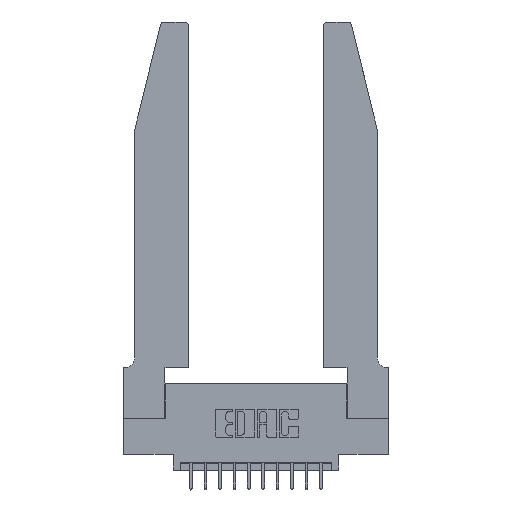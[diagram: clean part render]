
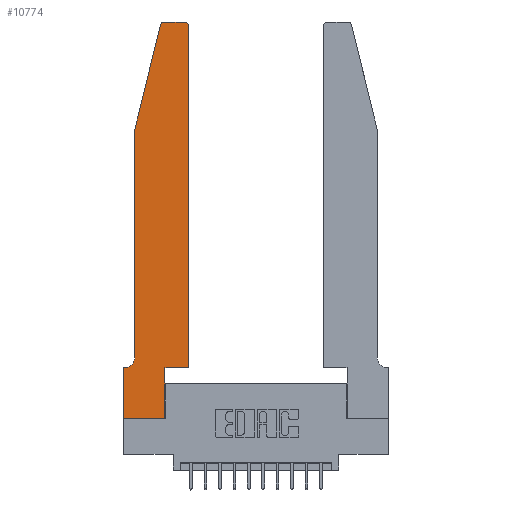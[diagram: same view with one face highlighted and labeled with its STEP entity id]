
A CAD part, top view. The second image highlights one B-rep face of the part: STEP entity #10774.
In plain terms, the highlighted planar face has unit normal (0, 0, 1).
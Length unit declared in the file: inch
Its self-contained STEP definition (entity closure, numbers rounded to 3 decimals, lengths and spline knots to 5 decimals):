
#90 = CARTESIAN_POINT ( 'NONE',  ( 0.0755, 2., 0.37 ) ) ;
#97 = CARTESIAN_POINT ( 'NONE',  ( 0.4505, 0.35, 0.37 ) ) ;
#165 = CIRCLE ( 'NONE', #15423, 0.07 ) ;
#335 = CARTESIAN_POINT ( 'NONE',  ( 0.0755, 0.42, 0.37 ) ) ;
#756 = VECTOR ( 'NONE', #4122, 39.37008 ) ;
#1157 = EDGE_CURVE ( 'NONE', #2570, #7950, #8377, .T. ) ;
#1395 = FACE_OUTER_BOUND ( 'NONE', #4094, .T. ) ;
#1536 = LINE ( 'NONE', #90, #12011 ) ;
#1605 = EDGE_CURVE ( 'NONE', #7950, #5005, #9120, .T. ) ;
#1927 = DIRECTION ( 'NONE',  ( 0., 0., -1. ) ) ;
#2083 = EDGE_CURVE ( 'NONE', #10482, #15649, #16942, .T. ) ;
#2090 = VERTEX_POINT ( 'NONE', #6530 ) ;
#2202 = AXIS2_PLACEMENT_3D ( 'NONE', #9430, #14817, #2800 ) ;
#2219 = CARTESIAN_POINT ( 'NONE',  ( 0.284, 2.75, 0.37 ) ) ;
#2226 = AXIS2_PLACEMENT_3D ( 'NONE', #7040, #16215, #12387 ) ;
#2570 = VERTEX_POINT ( 'NONE', #7397 ) ;
#2649 = CARTESIAN_POINT ( 'NONE',  ( 0.2605, 2.75, 0.37 ) ) ;
#2753 = VERTEX_POINT ( 'NONE', #16014 ) ;
#2800 = DIRECTION ( 'NONE',  ( 1., 0., 0. ) ) ;
#2968 = LINE ( 'NONE', #10841, #16239 ) ;
#3703 = AXIS2_PLACEMENT_3D ( 'NONE', #10741, #15989, #15657 ) ;
#3741 = ORIENTED_EDGE ( 'NONE', *, *, #15960, .T. ) ;
#3764 = VERTEX_POINT ( 'NONE', #15720 ) ;
#4094 = EDGE_LOOP ( 'NONE', ( #3741, #6626, #5440, #13302, #4902, #16029, #16630, #5879, #13497, #8921, #9785, #5282 ) ) ;
#4122 = DIRECTION ( 'NONE',  ( -1., 0., 0. ) ) ;
#4249 = VERTEX_POINT ( 'NONE', #335 ) ;
#4635 = CARTESIAN_POINT ( 'NONE',  ( 0., 0., 0.37 ) ) ;
#4716 = CIRCLE ( 'NONE', #2202, 0.03 ) ;
#4902 = ORIENTED_EDGE ( 'NONE', *, *, #15686, .T. ) ;
#5001 = LINE ( 'NONE', #10351, #11483 ) ;
#5005 = VERTEX_POINT ( 'NONE', #10716 ) ;
#5067 = CARTESIAN_POINT ( 'NONE',  ( 0.25487, 2.72718, 0.37 ) ) ;
#5282 = ORIENTED_EDGE ( 'NONE', *, *, #6026, .T. ) ;
#5380 = DIRECTION ( 'NONE',  ( 0., 1., 0. ) ) ;
#5440 = ORIENTED_EDGE ( 'NONE', *, *, #5965, .T. ) ;
#5478 = EDGE_CURVE ( 'NONE', #7269, #16284, #4716, .T. ) ;
#5767 = CARTESIAN_POINT ( 'NONE',  ( 0.2865, 0.35, 0.37 ) ) ;
#5879 = ORIENTED_EDGE ( 'NONE', *, *, #7337, .T. ) ;
#5965 = EDGE_CURVE ( 'NONE', #16284, #2090, #1536, .T. ) ;
#6026 = EDGE_CURVE ( 'NONE', #3764, #2753, #9749, .T. ) ;
#6442 = CARTESIAN_POINT ( 'NONE',  ( 0., 0., 0.37 ) ) ;
#6530 = CARTESIAN_POINT ( 'NONE',  ( 0.0755, 2., 0.37 ) ) ;
#6626 = ORIENTED_EDGE ( 'NONE', *, *, #5478, .T. ) ;
#7040 = CARTESIAN_POINT ( 'NONE',  ( 0.4205, 2.72, 0.37 ) ) ;
#7269 = VERTEX_POINT ( 'NONE', #2219 ) ;
#7337 = EDGE_CURVE ( 'NONE', #15649, #2570, #5001, .T. ) ;
#7397 = CARTESIAN_POINT ( 'NONE',  ( 0.2865, 0., 0.37 ) ) ;
#7950 = VERTEX_POINT ( 'NONE', #5767 ) ;
#8377 = LINE ( 'NONE', #13719, #16578 ) ;
#8412 = DIRECTION ( 'NONE',  ( -1., 0., 0. ) ) ;
#8921 = ORIENTED_EDGE ( 'NONE', *, *, #1605, .T. ) ;
#9120 = LINE ( 'NONE', #16748, #11090 ) ;
#9430 = CARTESIAN_POINT ( 'NONE',  ( 0.284, 2.72, 0.37 ) ) ;
#9749 = CIRCLE ( 'NONE', #2226, 0.03 ) ;
#9773 = CARTESIAN_POINT ( 'NONE',  ( 0.0055, 0.42, 0.37 ) ) ;
#9785 = ORIENTED_EDGE ( 'NONE', *, *, #14564, .T. ) ;
#10351 = CARTESIAN_POINT ( 'NONE',  ( 0., 0., 0.37 ) ) ;
#10473 = VECTOR ( 'NONE', #5380, 39.37008 ) ;
#10482 = VERTEX_POINT ( 'NONE', #14580 ) ;
#10716 = CARTESIAN_POINT ( 'NONE',  ( 0.4505, 0.35, 0.37 ) ) ;
#10741 = CARTESIAN_POINT ( 'NONE',  ( 0., 0.35, 0.37 ) ) ;
#10774 = ADVANCED_FACE ( 'NONE', ( #1395 ), #12069, .T. ) ;
#10786 = VERTEX_POINT ( 'NONE', #12240 ) ;
#10841 = CARTESIAN_POINT ( 'NONE',  ( 0.0755, 2., 0.37 ) ) ;
#11090 = VECTOR ( 'NONE', #12921, 39.37008 ) ;
#11272 = VECTOR ( 'NONE', #11799, 39.37008 ) ;
#11483 = VECTOR ( 'NONE', #14347, 39.37008 ) ;
#11799 = DIRECTION ( 'NONE',  ( 0., -1., 0. ) ) ;
#11956 = LINE ( 'NONE', #97, #10473 ) ;
#12011 = VECTOR ( 'NONE', #12216, 39.37008 ) ;
#12069 = PLANE ( 'NONE',  #3703 ) ;
#12216 = DIRECTION ( 'NONE',  ( -0.239, -0.971, 0. ) ) ;
#12240 = CARTESIAN_POINT ( 'NONE',  ( 0.0055, 0.35, 0.37 ) ) ;
#12387 = DIRECTION ( 'NONE',  ( 1., 0., 0. ) ) ;
#12539 = LINE ( 'NONE', #16544, #14882 ) ;
#12921 = DIRECTION ( 'NONE',  ( 1., 0., 0. ) ) ;
#13302 = ORIENTED_EDGE ( 'NONE', *, *, #15492, .T. ) ;
#13497 = ORIENTED_EDGE ( 'NONE', *, *, #1157, .T. ) ;
#13642 = DIRECTION ( 'NONE',  ( 0., -1., 0. ) ) ;
#13719 = CARTESIAN_POINT ( 'NONE',  ( 0.2865, 0.35, 0.37 ) ) ;
#14347 = DIRECTION ( 'NONE',  ( 1., 0., 0. ) ) ;
#14564 = EDGE_CURVE ( 'NONE', #5005, #3764, #11956, .T. ) ;
#14580 = CARTESIAN_POINT ( 'NONE',  ( 0., 0.35, 0.37 ) ) ;
#14817 = DIRECTION ( 'NONE',  ( 0., 0., 1. ) ) ;
#14882 = VECTOR ( 'NONE', #8412, 39.37008 ) ;
#15067 = DIRECTION ( 'NONE',  ( -1., 0., 0. ) ) ;
#15132 = DIRECTION ( 'NONE',  ( 0., 1., 0. ) ) ;
#15423 = AXIS2_PLACEMENT_3D ( 'NONE', #9773, #1927, #15067 ) ;
#15492 = EDGE_CURVE ( 'NONE', #2090, #4249, #2968, .T. ) ;
#15649 = VERTEX_POINT ( 'NONE', #4635 ) ;
#15657 = DIRECTION ( 'NONE',  ( 1., 0., 0. ) ) ;
#15686 = EDGE_CURVE ( 'NONE', #4249, #10786, #165, .T. ) ;
#15720 = CARTESIAN_POINT ( 'NONE',  ( 0.4505, 2.72, 0.37 ) ) ;
#15960 = EDGE_CURVE ( 'NONE', #2753, #7269, #16025, .T. ) ;
#15989 = DIRECTION ( 'NONE',  ( 0., 0., 1. ) ) ;
#16014 = CARTESIAN_POINT ( 'NONE',  ( 0.4205, 2.75, 0.37 ) ) ;
#16025 = LINE ( 'NONE', #2649, #756 ) ;
#16029 = ORIENTED_EDGE ( 'NONE', *, *, #16094, .T. ) ;
#16094 = EDGE_CURVE ( 'NONE', #10786, #10482, #12539, .T. ) ;
#16215 = DIRECTION ( 'NONE',  ( 0., 0., 1. ) ) ;
#16239 = VECTOR ( 'NONE', #13642, 39.37008 ) ;
#16284 = VERTEX_POINT ( 'NONE', #5067 ) ;
#16544 = CARTESIAN_POINT ( 'NONE',  ( 0.0755, 0.35, 0.37 ) ) ;
#16578 = VECTOR ( 'NONE', #15132, 39.37008 ) ;
#16630 = ORIENTED_EDGE ( 'NONE', *, *, #2083, .T. ) ;
#16748 = CARTESIAN_POINT ( 'NONE',  ( 0.4505, 0.35, 0.37 ) ) ;
#16942 = LINE ( 'NONE', #6442, #11272 ) ;
